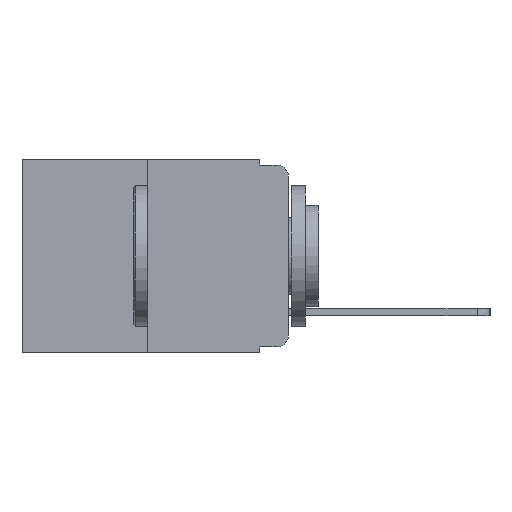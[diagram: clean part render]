
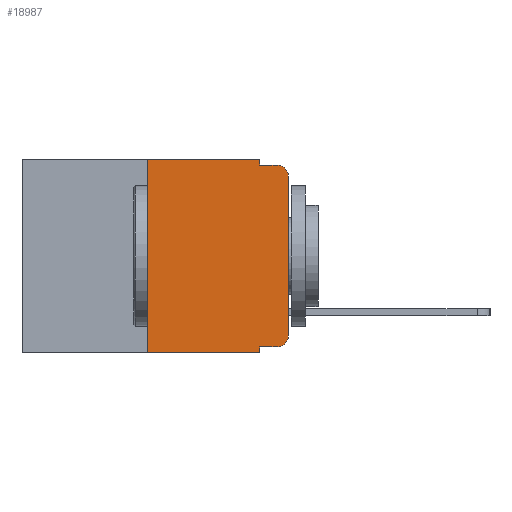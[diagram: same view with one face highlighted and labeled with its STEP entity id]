
A CAD part, left-side view. The second image highlights one B-rep face of the part: STEP entity #18987.
In plain terms, the highlighted planar face has unit normal (-1, 0, 0).
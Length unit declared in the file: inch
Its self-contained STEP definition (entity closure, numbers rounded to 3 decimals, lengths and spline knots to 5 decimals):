
#143 = LINE ( 'NONE', #18971, #19543 ) ;
#380 = VERTEX_POINT ( 'NONE', #18532 ) ;
#435 = VECTOR ( 'NONE', #5081, 39.37008 ) ;
#672 = ORIENTED_EDGE ( 'NONE', *, *, #17729, .F. ) ;
#723 = DIRECTION ( 'NONE',  ( 0., 0., -1. ) ) ;
#976 = AXIS2_PLACEMENT_3D ( 'NONE', #16165, #4863, #18059 ) ;
#1728 = CARTESIAN_POINT ( 'NONE',  ( 0., 0.051, 0. ) ) ;
#1814 = ORIENTED_EDGE ( 'NONE', *, *, #15513, .T. ) ;
#1996 = VECTOR ( 'NONE', #21349, 39.37008 ) ;
#2083 = ORIENTED_EDGE ( 'NONE', *, *, #20242, .T. ) ;
#2588 = LINE ( 'NONE', #6189, #1996 ) ;
#3993 = DIRECTION ( 'NONE',  ( -1., 0., 0. ) ) ;
#4271 = LINE ( 'NONE', #7307, #9199 ) ;
#4754 = CARTESIAN_POINT ( 'NONE',  ( 0., 0.051, -0.333 ) ) ;
#4863 = DIRECTION ( 'NONE',  ( -1., 0., 0. ) ) ;
#5081 = DIRECTION ( 'NONE',  ( 0., 0., -1. ) ) ;
#5764 = CARTESIAN_POINT ( 'NONE',  ( 0., 0., -0.03 ) ) ;
#6092 = VERTEX_POINT ( 'NONE', #15486 ) ;
#6123 = CARTESIAN_POINT ( 'NONE',  ( 0., 0.02, -0.333 ) ) ;
#6189 = CARTESIAN_POINT ( 'NONE',  ( 0., 0.051, -0.333 ) ) ;
#6729 = CARTESIAN_POINT ( 'NONE',  ( 0., 0.25, 0. ) ) ;
#6868 = CARTESIAN_POINT ( 'NONE',  ( 0., 0.051, 0. ) ) ;
#7045 = ORIENTED_EDGE ( 'NONE', *, *, #10113, .T. ) ;
#7307 = CARTESIAN_POINT ( 'NONE',  ( 0., 0., 0. ) ) ;
#7401 = LINE ( 'NONE', #14301, #23123 ) ;
#7528 = CIRCLE ( 'NONE', #23781, 0.02 ) ;
#7545 = EDGE_CURVE ( 'NONE', #19710, #380, #19797, .T. ) ;
#7775 = VECTOR ( 'NONE', #21913, 39.37008 ) ;
#8813 = CARTESIAN_POINT ( 'NONE',  ( 0., 0.25, 0. ) ) ;
#9199 = VECTOR ( 'NONE', #11124, 39.37008 ) ;
#9495 = VECTOR ( 'NONE', #12634, 39.37008 ) ;
#10113 = EDGE_CURVE ( 'NONE', #11243, #19710, #2588, .T. ) ;
#10298 = EDGE_CURVE ( 'NONE', #19148, #16330, #17869, .T. ) ;
#10856 = ORIENTED_EDGE ( 'NONE', *, *, #10298, .F. ) ;
#11124 = DIRECTION ( 'NONE',  ( 0., 0., 1. ) ) ;
#11243 = VERTEX_POINT ( 'NONE', #4754 ) ;
#11887 = DIRECTION ( 'NONE',  ( 1., 0., 0. ) ) ;
#12436 = ORIENTED_EDGE ( 'NONE', *, *, #7545, .T. ) ;
#12625 = EDGE_CURVE ( 'NONE', #11243, #21192, #20383, .T. ) ;
#12634 = DIRECTION ( 'NONE',  ( 0., 0., 1. ) ) ;
#14207 = EDGE_LOOP ( 'NONE', ( #17938, #2083, #672, #17978, #10856, #18859, #1814, #17408, #7045, #12436 ) ) ;
#14301 = CARTESIAN_POINT ( 'NONE',  ( 0., 0.473, -0.343 ) ) ;
#15167 = EDGE_CURVE ( 'NONE', #6092, #19148, #19607, .T. ) ;
#15262 = CARTESIAN_POINT ( 'NONE',  ( 0., 0.02, -0.03 ) ) ;
#15365 = CARTESIAN_POINT ( 'NONE',  ( 0., 0.051, -0.01 ) ) ;
#15422 = CARTESIAN_POINT ( 'NONE',  ( 0., 0.02, -0.01 ) ) ;
#15486 = CARTESIAN_POINT ( 'NONE',  ( 0., 0.25, -0.343 ) ) ;
#15513 = EDGE_CURVE ( 'NONE', #6092, #21192, #7401, .T. ) ;
#15789 = VECTOR ( 'NONE', #16387, 39.37008 ) ;
#16165 = CARTESIAN_POINT ( 'NONE',  ( 0., 0.02, -0.313 ) ) ;
#16217 = DIRECTION ( 'NONE',  ( 0., -1., 0. ) ) ;
#16330 = VERTEX_POINT ( 'NONE', #1728 ) ;
#16372 = LINE ( 'NONE', #20183, #15789 ) ;
#16387 = DIRECTION ( 'NONE',  ( 0., -1., 0. ) ) ;
#16446 = EDGE_CURVE ( 'NONE', #16330, #18879, #143, .T. ) ;
#17161 = DIRECTION ( 'NONE',  ( 0., 0., -1. ) ) ;
#17408 = ORIENTED_EDGE ( 'NONE', *, *, #12625, .F. ) ;
#17523 = CARTESIAN_POINT ( 'NONE',  ( 0., 0.473, 0. ) ) ;
#17729 = EDGE_CURVE ( 'NONE', #18879, #23849, #16372, .T. ) ;
#17869 = LINE ( 'NONE', #20010, #7775 ) ;
#17938 = ORIENTED_EDGE ( 'NONE', *, *, #21548, .T. ) ;
#17978 = ORIENTED_EDGE ( 'NONE', *, *, #16446, .F. ) ;
#18059 = DIRECTION ( 'NONE',  ( 0., 0., -1. ) ) ;
#18061 = AXIS2_PLACEMENT_3D ( 'NONE', #17523, #11887, #723 ) ;
#18532 = CARTESIAN_POINT ( 'NONE',  ( 0., 0., -0.313 ) ) ;
#18859 = ORIENTED_EDGE ( 'NONE', *, *, #15167, .F. ) ;
#18879 = VERTEX_POINT ( 'NONE', #15365 ) ;
#18971 = CARTESIAN_POINT ( 'NONE',  ( 0., 0.051, 0. ) ) ;
#18987 = ADVANCED_FACE ( 'NONE', ( #21355 ), #21335, .F. ) ;
#19148 = VERTEX_POINT ( 'NONE', #6729 ) ;
#19539 = CARTESIAN_POINT ( 'NONE',  ( 0., 0.051, -0.343 ) ) ;
#19543 = VECTOR ( 'NONE', #22769, 39.37008 ) ;
#19607 = LINE ( 'NONE', #8813, #9495 ) ;
#19710 = VERTEX_POINT ( 'NONE', #6123 ) ;
#19797 = CIRCLE ( 'NONE', #976, 0.02 ) ;
#20010 = CARTESIAN_POINT ( 'NONE',  ( 0., 0.473, 0. ) ) ;
#20183 = CARTESIAN_POINT ( 'NONE',  ( 0., 0.051, -0.01 ) ) ;
#20218 = VERTEX_POINT ( 'NONE', #5764 ) ;
#20242 = EDGE_CURVE ( 'NONE', #20218, #23849, #7528, .T. ) ;
#20383 = LINE ( 'NONE', #6868, #435 ) ;
#21192 = VERTEX_POINT ( 'NONE', #19539 ) ;
#21335 = PLANE ( 'NONE',  #18061 ) ;
#21349 = DIRECTION ( 'NONE',  ( 0., -1., 0. ) ) ;
#21355 = FACE_OUTER_BOUND ( 'NONE', #14207, .T. ) ;
#21548 = EDGE_CURVE ( 'NONE', #380, #20218, #4271, .T. ) ;
#21913 = DIRECTION ( 'NONE',  ( 0., -1., 0. ) ) ;
#22769 = DIRECTION ( 'NONE',  ( 0., 0., -1. ) ) ;
#23123 = VECTOR ( 'NONE', #16217, 39.37008 ) ;
#23781 = AXIS2_PLACEMENT_3D ( 'NONE', #15262, #3993, #17161 ) ;
#23849 = VERTEX_POINT ( 'NONE', #15422 ) ;
